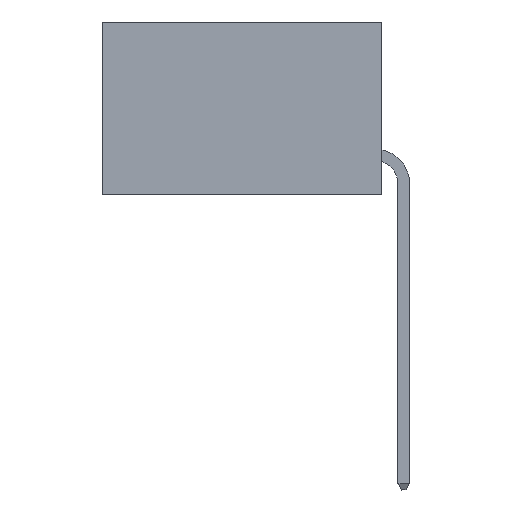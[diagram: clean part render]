
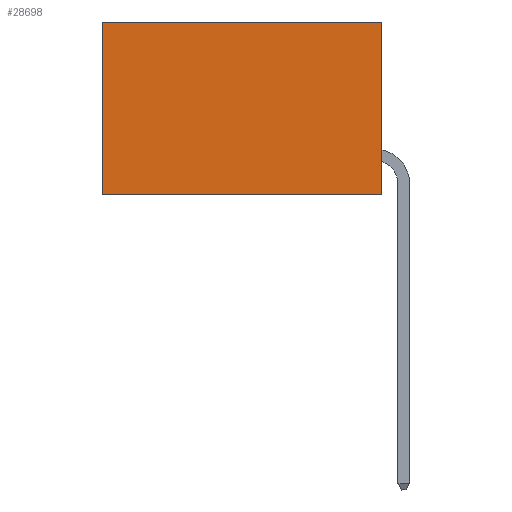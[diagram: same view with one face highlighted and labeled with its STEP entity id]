
A CAD part, left-side view. The second image highlights one B-rep face of the part: STEP entity #28698.
In plain terms, the highlighted planar face has unit normal (-1, 0, 0).
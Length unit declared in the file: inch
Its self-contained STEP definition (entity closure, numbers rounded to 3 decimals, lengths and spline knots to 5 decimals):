
#118 = CARTESIAN_POINT ( 'NONE',  ( 0.2875, 0., 0. ) ) ;
#1038 = CARTESIAN_POINT ( 'NONE',  ( 0.2875, 0., -0.37 ) ) ;
#1245 = LINE ( 'NONE', #25155, #15749 ) ;
#2288 = EDGE_LOOP ( 'NONE', ( #26826, #11327, #3336, #4625 ) ) ;
#3336 = ORIENTED_EDGE ( 'NONE', *, *, #4309, .F. ) ;
#4309 = EDGE_CURVE ( 'NONE', #24655, #4440, #25989, .T. ) ;
#4440 = VERTEX_POINT ( 'NONE', #1038 ) ;
#4571 = VECTOR ( 'NONE', #23912, 39.37008 ) ;
#4625 = ORIENTED_EDGE ( 'NONE', *, *, #10248, .T. ) ;
#4819 = CARTESIAN_POINT ( 'NONE',  ( 0.2875, 0., -0.37 ) ) ;
#5452 = VECTOR ( 'NONE', #16546, 39.37008 ) ;
#6447 = DIRECTION ( 'NONE',  ( 1., 0., 0. ) ) ;
#7931 = LINE ( 'NONE', #4819, #4571 ) ;
#8029 = LINE ( 'NONE', #26927, #30721 ) ;
#8258 = DIRECTION ( 'NONE',  ( 0., 1., 0. ) ) ;
#9969 = EDGE_CURVE ( 'NONE', #4440, #13203, #7931, .T. ) ;
#10206 = FACE_OUTER_BOUND ( 'NONE', #2288, .T. ) ;
#10248 = EDGE_CURVE ( 'NONE', #24655, #18968, #1245, .T. ) ;
#11327 = ORIENTED_EDGE ( 'NONE', *, *, #9969, .F. ) ;
#13203 = VERTEX_POINT ( 'NONE', #28575 ) ;
#13332 = PLANE ( 'NONE',  #14874 ) ;
#14874 = AXIS2_PLACEMENT_3D ( 'NONE', #27802, #6447, #22841 ) ;
#15749 = VECTOR ( 'NONE', #8258, 39.37008 ) ;
#16546 = DIRECTION ( 'NONE',  ( 0., 0., -1. ) ) ;
#18968 = VERTEX_POINT ( 'NONE', #28749 ) ;
#21841 = EDGE_CURVE ( 'NONE', #18968, #13203, #8029, .T. ) ;
#22841 = DIRECTION ( 'NONE',  ( 0., 0., -1. ) ) ;
#23912 = DIRECTION ( 'NONE',  ( 0., 1., 0. ) ) ;
#24437 = DIRECTION ( 'NONE',  ( 0., 0., -1. ) ) ;
#24655 = VERTEX_POINT ( 'NONE', #118 ) ;
#25155 = CARTESIAN_POINT ( 'NONE',  ( 0.2875, 0., 0. ) ) ;
#25989 = LINE ( 'NONE', #30769, #5452 ) ;
#26826 = ORIENTED_EDGE ( 'NONE', *, *, #21841, .T. ) ;
#26927 = CARTESIAN_POINT ( 'NONE',  ( 0.2875, 0.6, 0. ) ) ;
#27802 = CARTESIAN_POINT ( 'NONE',  ( 0.2875, 0., 0. ) ) ;
#28575 = CARTESIAN_POINT ( 'NONE',  ( 0.2875, 0.6, -0.37 ) ) ;
#28698 = ADVANCED_FACE ( 'NONE', ( #10206 ), #13332, .F. ) ;
#28749 = CARTESIAN_POINT ( 'NONE',  ( 0.2875, 0.6, 0. ) ) ;
#30721 = VECTOR ( 'NONE', #24437, 39.37008 ) ;
#30769 = CARTESIAN_POINT ( 'NONE',  ( 0.2875, 0., 0. ) ) ;
